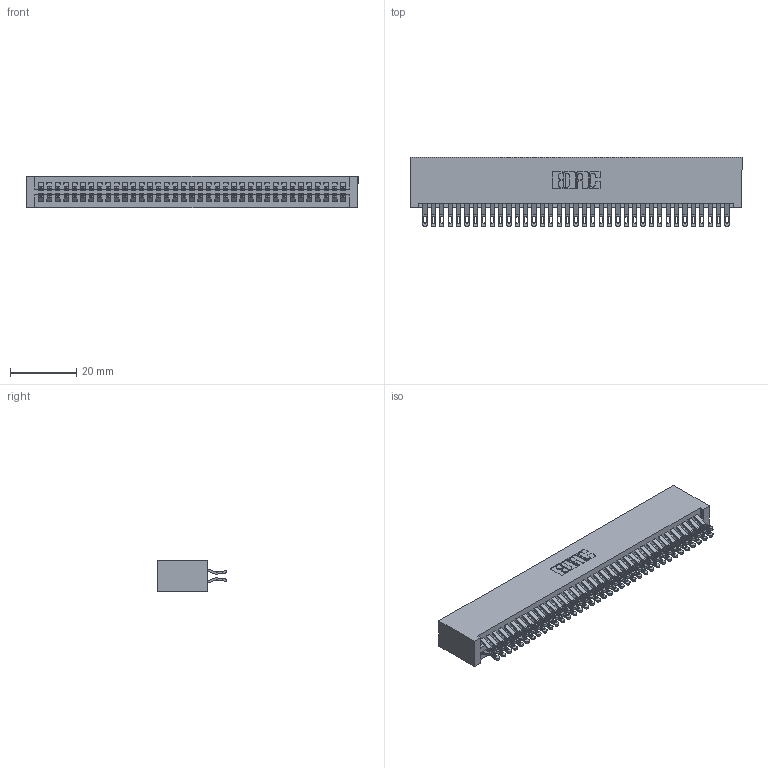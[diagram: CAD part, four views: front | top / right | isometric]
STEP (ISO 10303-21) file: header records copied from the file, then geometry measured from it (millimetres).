
FILE_DESCRIPTION (( 'STEP AP203' ), '1' );
FILE_NAME ('345-074-555-201.STEP', '2018-10-02T13:10:28', ( '' ), ( '' ), 'SwSTEP 2.0', 'SolidWorks 2016', '' );
FILE_SCHEMA (( 'CONFIG_CONTROL_DESIGN' ));
Length unit declared in the file: inch
Products named in the file (3): 345 Part_No Mounting Lugs; 345-074-555-201; 345-292-001_555 Tail
Assembly tree (75 placements, depth 2):
  345-074-555-201
    345 Part_No Mounting Lugs
    345-292-001_555 Tail  x74
Bounding box: 100.58 x 21.13 x 9.4 mm (x, y, z)
Volume: 10555 mm3; surface area: 16555 mm2
Topology: 75 solids, 75 shells, 4262 faces, 13415 edges, 8942 vertices
Faces by surface type: plane 2370, cylinder 1892
Entity records: 29753 total; most frequent: CARTESIAN_POINT 5026, ORIENTED_EDGE 4930, DIRECTION 4401, EDGE_CURVE 2465, VECTOR 2173, LINE 2173, VERTEX_POINT 1642, AXIS2_PLACEMENT_3D 1114
